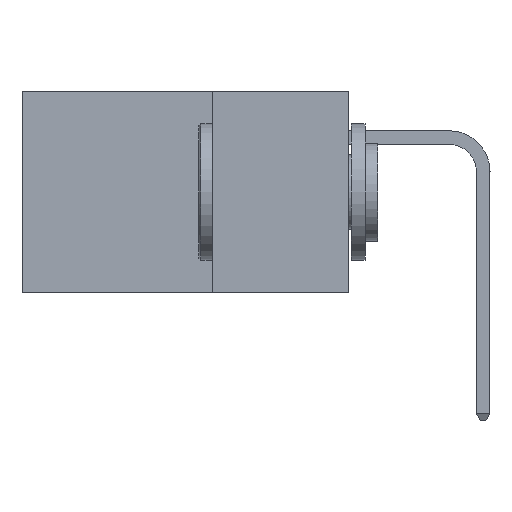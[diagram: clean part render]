
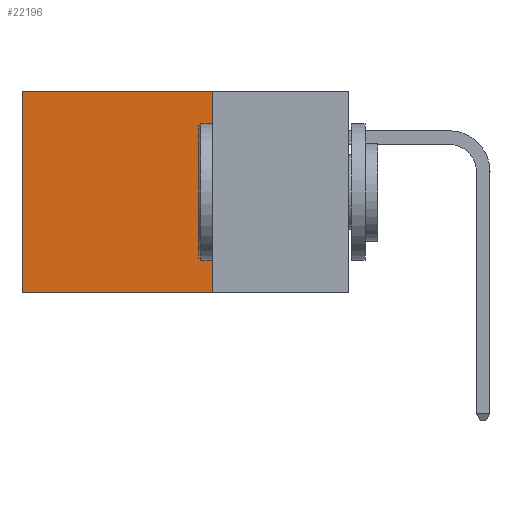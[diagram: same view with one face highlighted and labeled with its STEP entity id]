
A CAD part, left-side view. The second image highlights one B-rep face of the part: STEP entity #22196.
In plain terms, the highlighted planar face has unit normal (-1, 0, 0).
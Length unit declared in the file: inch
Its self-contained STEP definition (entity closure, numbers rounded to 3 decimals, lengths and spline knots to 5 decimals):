
#517 = DIRECTION ( 'NONE',  ( 0., 1., 0. ) ) ;
#2562 = VERTEX_POINT ( 'NONE', #27762 ) ;
#2753 = ORIENTED_EDGE ( 'NONE', *, *, #7774, .T. ) ;
#4001 = AXIS2_PLACEMENT_3D ( 'NONE', #23142, #4323, #26230 ) ;
#4300 = EDGE_CURVE ( 'NONE', #13293, #9631, #13341, .T. ) ;
#4323 = DIRECTION ( 'NONE',  ( 1., 0., 0. ) ) ;
#4350 = CARTESIAN_POINT ( 'NONE',  ( 0.2875, 0.6, -0.37 ) ) ;
#5326 = CARTESIAN_POINT ( 'NONE',  ( 0.2875, 0.25, 0. ) ) ;
#7774 = EDGE_CURVE ( 'NONE', #9631, #15625, #10108, .T. ) ;
#9631 = VERTEX_POINT ( 'NONE', #17335 ) ;
#10108 = LINE ( 'NONE', #14830, #17476 ) ;
#10737 = LINE ( 'NONE', #5326, #33634 ) ;
#11121 = CARTESIAN_POINT ( 'NONE',  ( 0.2875, 0.25, -0.37 ) ) ;
#11923 = ORIENTED_EDGE ( 'NONE', *, *, #34123, .F. ) ;
#12150 = EDGE_LOOP ( 'NONE', ( #2753, #29293, #11923, #13189 ) ) ;
#12350 = VECTOR ( 'NONE', #517, 39.37008 ) ;
#12689 = VECTOR ( 'NONE', #14290, 39.37008 ) ;
#13189 = ORIENTED_EDGE ( 'NONE', *, *, #4300, .T. ) ;
#13293 = VERTEX_POINT ( 'NONE', #32565 ) ;
#13341 = LINE ( 'NONE', #37844, #12350 ) ;
#14290 = DIRECTION ( 'NONE',  ( 0., 1., 0. ) ) ;
#14830 = CARTESIAN_POINT ( 'NONE',  ( 0.2875, 0.6, 0. ) ) ;
#15625 = VERTEX_POINT ( 'NONE', #4350 ) ;
#16853 = PLANE ( 'NONE',  #4001 ) ;
#17335 = CARTESIAN_POINT ( 'NONE',  ( 0.2875, 0.6, 0. ) ) ;
#17476 = VECTOR ( 'NONE', #30473, 39.37008 ) ;
#19651 = FACE_OUTER_BOUND ( 'NONE', #12150, .T. ) ;
#21076 = LINE ( 'NONE', #11121, #12689 ) ;
#22196 = ADVANCED_FACE ( 'NONE', ( #19651 ), #16853, .F. ) ;
#23142 = CARTESIAN_POINT ( 'NONE',  ( 0.2875, 0.25, 0. ) ) ;
#26230 = DIRECTION ( 'NONE',  ( 0., 0., -1. ) ) ;
#27762 = CARTESIAN_POINT ( 'NONE',  ( 0.2875, 0.25, -0.37 ) ) ;
#29293 = ORIENTED_EDGE ( 'NONE', *, *, #34062, .F. ) ;
#30326 = DIRECTION ( 'NONE',  ( 0., 0., -1. ) ) ;
#30473 = DIRECTION ( 'NONE',  ( 0., 0., -1. ) ) ;
#32565 = CARTESIAN_POINT ( 'NONE',  ( 0.2875, 0.25, 0. ) ) ;
#33634 = VECTOR ( 'NONE', #30326, 39.37008 ) ;
#34062 = EDGE_CURVE ( 'NONE', #2562, #15625, #21076, .T. ) ;
#34123 = EDGE_CURVE ( 'NONE', #13293, #2562, #10737, .T. ) ;
#37844 = CARTESIAN_POINT ( 'NONE',  ( 0.2875, 0.25, 0. ) ) ;
